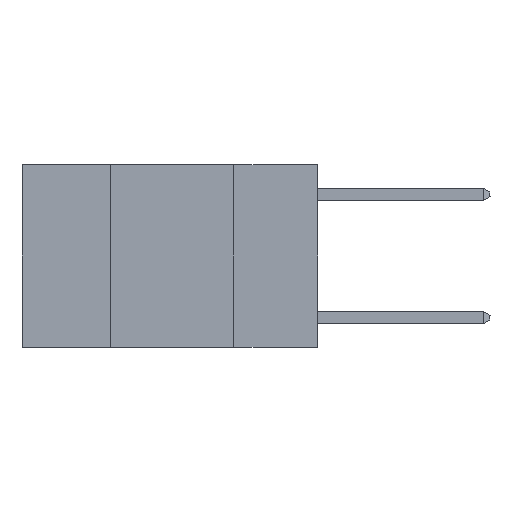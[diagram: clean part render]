
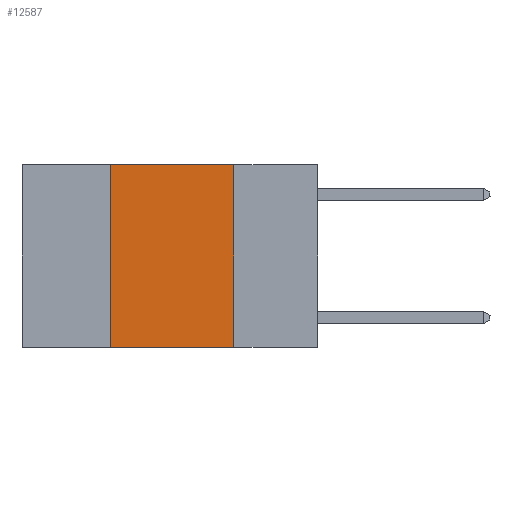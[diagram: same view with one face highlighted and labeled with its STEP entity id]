
A CAD part, left-side view. The second image highlights one B-rep face of the part: STEP entity #12587.
In plain terms, the highlighted planar face has unit normal (-1, 0, 0).
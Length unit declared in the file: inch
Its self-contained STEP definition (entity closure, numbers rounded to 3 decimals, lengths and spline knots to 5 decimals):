
#368 = CARTESIAN_POINT ( 'NONE',  ( 0., 0.6, -0.37 ) ) ;
#2250 = VERTEX_POINT ( 'NONE', #12138 ) ;
#2932 = FACE_OUTER_BOUND ( 'NONE', #8953, .T. ) ;
#3476 = CARTESIAN_POINT ( 'NONE',  ( 0., 0.42, 0. ) ) ;
#4354 = VERTEX_POINT ( 'NONE', #6559 ) ;
#5171 = CARTESIAN_POINT ( 'NONE',  ( 0., 0.17, 0. ) ) ;
#5357 = LINE ( 'NONE', #9775, #14691 ) ;
#6559 = CARTESIAN_POINT ( 'NONE',  ( 0., 0.17, -0.37 ) ) ;
#6949 = EDGE_CURVE ( 'NONE', #16521, #2250, #13346, .T. ) ;
#7158 = AXIS2_PLACEMENT_3D ( 'NONE', #12287, #10776, #9056 ) ;
#7188 = CARTESIAN_POINT ( 'NONE',  ( 0., 0.17, 0. ) ) ;
#7955 = VECTOR ( 'NONE', #11592, 39.37008 ) ;
#8372 = LINE ( 'NONE', #368, #7955 ) ;
#8770 = LINE ( 'NONE', #7188, #13817 ) ;
#8953 = EDGE_LOOP ( 'NONE', ( #17336, #9592, #9319, #19254 ) ) ;
#9056 = DIRECTION ( 'NONE',  ( 0., 0., -1. ) ) ;
#9319 = ORIENTED_EDGE ( 'NONE', *, *, #6949, .F. ) ;
#9320 = CARTESIAN_POINT ( 'NONE',  ( 0., 0.42, -0.37 ) ) ;
#9592 = ORIENTED_EDGE ( 'NONE', *, *, #14559, .F. ) ;
#9775 = CARTESIAN_POINT ( 'NONE',  ( 0., 0.6, 0. ) ) ;
#10776 = DIRECTION ( 'NONE',  ( 1., 0., 0. ) ) ;
#11592 = DIRECTION ( 'NONE',  ( 0., -1., 0. ) ) ;
#12138 = CARTESIAN_POINT ( 'NONE',  ( 0., 0.42, 0. ) ) ;
#12287 = CARTESIAN_POINT ( 'NONE',  ( 0., 0.6, 0. ) ) ;
#12587 = ADVANCED_FACE ( 'NONE', ( #2932 ), #15661, .F. ) ;
#13124 = DIRECTION ( 'NONE',  ( 0., -1., 0. ) ) ;
#13346 = LINE ( 'NONE', #3476, #19402 ) ;
#13817 = VECTOR ( 'NONE', #20019, 39.37008 ) ;
#14559 = EDGE_CURVE ( 'NONE', #2250, #17127, #5357, .T. ) ;
#14691 = VECTOR ( 'NONE', #13124, 39.37008 ) ;
#15661 = PLANE ( 'NONE',  #7158 ) ;
#16521 = VERTEX_POINT ( 'NONE', #9320 ) ;
#17127 = VERTEX_POINT ( 'NONE', #5171 ) ;
#17336 = ORIENTED_EDGE ( 'NONE', *, *, #20704, .F. ) ;
#17963 = DIRECTION ( 'NONE',  ( 0., 0., 1. ) ) ;
#18136 = EDGE_CURVE ( 'NONE', #16521, #4354, #8372, .T. ) ;
#19254 = ORIENTED_EDGE ( 'NONE', *, *, #18136, .T. ) ;
#19402 = VECTOR ( 'NONE', #17963, 39.37008 ) ;
#20019 = DIRECTION ( 'NONE',  ( 0., 0., -1. ) ) ;
#20704 = EDGE_CURVE ( 'NONE', #17127, #4354, #8770, .T. ) ;
